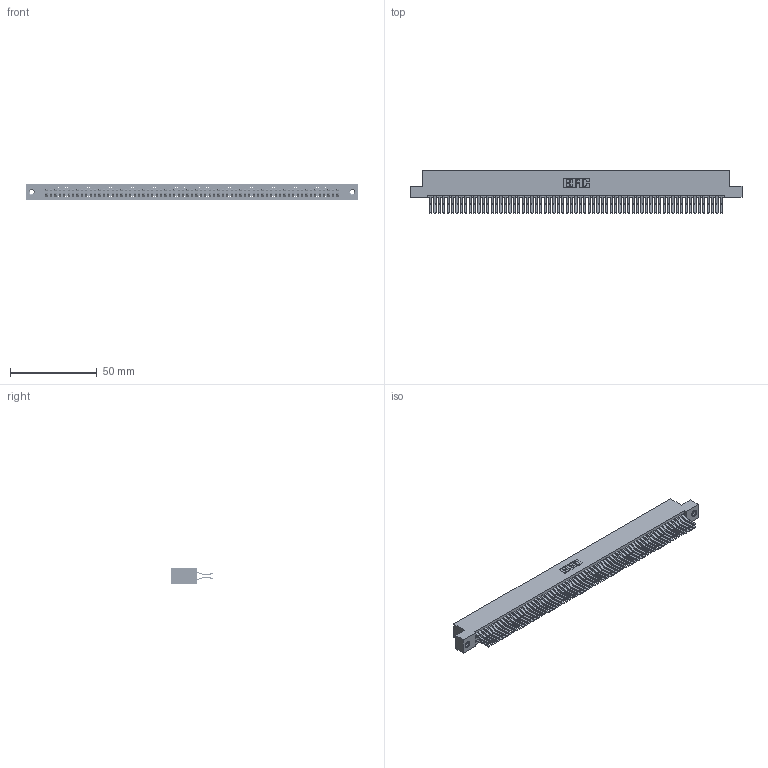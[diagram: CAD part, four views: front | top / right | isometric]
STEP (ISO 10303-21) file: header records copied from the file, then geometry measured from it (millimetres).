
FILE_DESCRIPTION (( 'STEP AP203' ), '1' );
FILE_NAME ('345-134-560-208.STEP', '2019-11-08T05:17:39', ( '' ), ( '' ), 'SwSTEP 2.0', 'SolidWorks 2016', '' );
FILE_SCHEMA (( 'CONFIG_CONTROL_DESIGN' ));
Length unit declared in the file: inch
Products named in the file (4): 345-292-001_560 Tail; 345-250-001_345-250-003-102; 345-134-560-208; 345 Part_Flush Mounting Lugs - 0.156 Dia-TI
Assembly tree (137 placements, depth 2):
  345-134-560-208
    345 Part_Flush Mounting Lugs - 0.156 Dia-TI
    345-292-001_560 Tail  x134
    345-250-001_345-250-003-102  x2
Bounding box: 191.39 x 24.45 x 9.4 mm (x, y, z)
Volume: 19695.6 mm3; surface area: 31869.9 mm2
Topology: 137 solids, 137 shells, 7154 faces, 21247 edges, 13978 vertices
Faces by surface type: plane 4534, cylinder 2604, cone 12, torus 4
Entity records: 50478 total; most frequent: CARTESIAN_POINT 8419, ORIENTED_EDGE 8346, DIRECTION 7423, EDGE_CURVE 4173, VECTOR 3749, LINE 3749, VERTEX_POINT 2776, AXIS2_PLACEMENT_3D 1837
